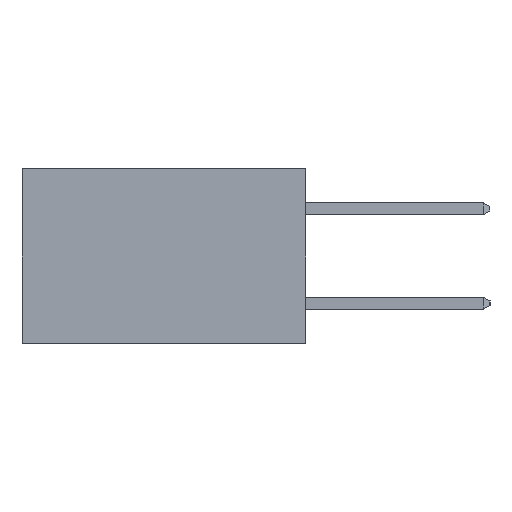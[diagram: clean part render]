
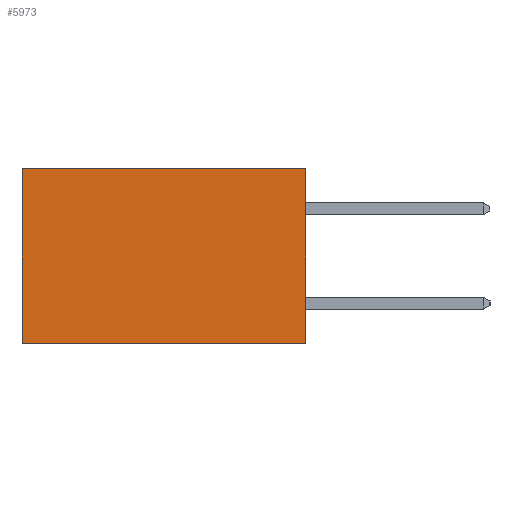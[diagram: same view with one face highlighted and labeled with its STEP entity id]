
A CAD part, left-side view. The second image highlights one B-rep face of the part: STEP entity #5973.
In plain terms, the highlighted planar face has unit normal (-1, 0, 0).
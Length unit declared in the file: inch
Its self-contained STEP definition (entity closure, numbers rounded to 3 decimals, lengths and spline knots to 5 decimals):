
#150 = CARTESIAN_POINT ( 'NONE',  ( 0.2615, 0., 0. ) ) ;
#234 = LINE ( 'NONE', #10701, #11883 ) ;
#260 = DIRECTION ( 'NONE',  ( 0., 1., 0. ) ) ;
#1570 = LINE ( 'NONE', #11582, #7131 ) ;
#1849 = LINE ( 'NONE', #150, #4543 ) ;
#2725 = AXIS2_PLACEMENT_3D ( 'NONE', #12307, #11681, #11659 ) ;
#3137 = VERTEX_POINT ( 'NONE', #5452 ) ;
#3996 = VECTOR ( 'NONE', #7369, 39.37008 ) ;
#4543 = VECTOR ( 'NONE', #260, 39.37008 ) ;
#4734 = EDGE_CURVE ( 'NONE', #9294, #6359, #234, .T. ) ;
#5164 = CARTESIAN_POINT ( 'NONE',  ( 0.2615, 0., -0.37 ) ) ;
#5378 = EDGE_LOOP ( 'NONE', ( #11244, #5921, #7573, #13435 ) ) ;
#5452 = CARTESIAN_POINT ( 'NONE',  ( 0.2615, 0., 0. ) ) ;
#5631 = EDGE_CURVE ( 'NONE', #10589, #6359, #9439, .T. ) ;
#5921 = ORIENTED_EDGE ( 'NONE', *, *, #5631, .F. ) ;
#5973 = ADVANCED_FACE ( 'NONE', ( #13690 ), #11724, .F. ) ;
#6359 = VERTEX_POINT ( 'NONE', #10656 ) ;
#7131 = VECTOR ( 'NONE', #11550, 39.37008 ) ;
#7369 = DIRECTION ( 'NONE',  ( 0., 1., 0. ) ) ;
#7573 = ORIENTED_EDGE ( 'NONE', *, *, #9505, .F. ) ;
#9087 = CARTESIAN_POINT ( 'NONE',  ( 0.2615, 0., -0.37 ) ) ;
#9294 = VERTEX_POINT ( 'NONE', #12913 ) ;
#9439 = LINE ( 'NONE', #9087, #3996 ) ;
#9505 = EDGE_CURVE ( 'NONE', #3137, #10589, #1570, .T. ) ;
#10589 = VERTEX_POINT ( 'NONE', #5164 ) ;
#10656 = CARTESIAN_POINT ( 'NONE',  ( 0.2615, 0.6, -0.37 ) ) ;
#10701 = CARTESIAN_POINT ( 'NONE',  ( 0.2615, 0.6, -0.37 ) ) ;
#11244 = ORIENTED_EDGE ( 'NONE', *, *, #4734, .T. ) ;
#11550 = DIRECTION ( 'NONE',  ( 0., 0., -1. ) ) ;
#11582 = CARTESIAN_POINT ( 'NONE',  ( 0.2615, 0., -0.37 ) ) ;
#11659 = DIRECTION ( 'NONE',  ( 0., 0., -1. ) ) ;
#11681 = DIRECTION ( 'NONE',  ( 1., 0., 0. ) ) ;
#11724 = PLANE ( 'NONE',  #2725 ) ;
#11883 = VECTOR ( 'NONE', #13641, 39.37008 ) ;
#12307 = CARTESIAN_POINT ( 'NONE',  ( 0.2615, 0., -0.37 ) ) ;
#12698 = EDGE_CURVE ( 'NONE', #3137, #9294, #1849, .T. ) ;
#12913 = CARTESIAN_POINT ( 'NONE',  ( 0.2615, 0.6, 0. ) ) ;
#13435 = ORIENTED_EDGE ( 'NONE', *, *, #12698, .T. ) ;
#13641 = DIRECTION ( 'NONE',  ( 0., 0., -1. ) ) ;
#13690 = FACE_OUTER_BOUND ( 'NONE', #5378, .T. ) ;
